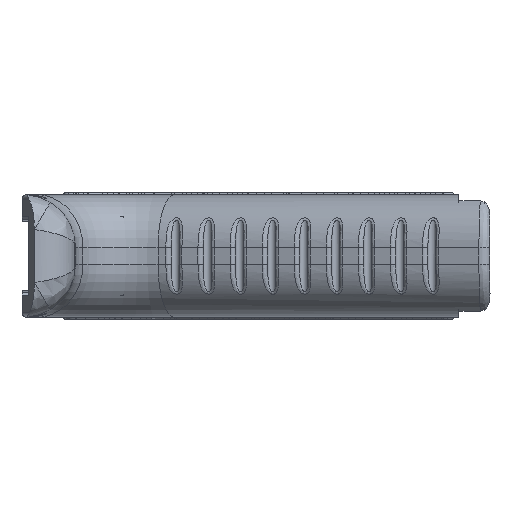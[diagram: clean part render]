
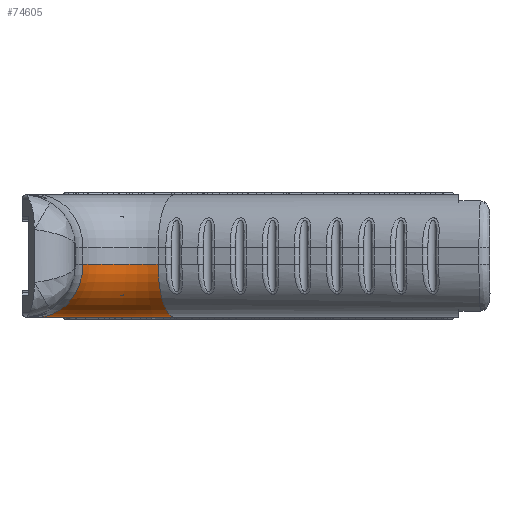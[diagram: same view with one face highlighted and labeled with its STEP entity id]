
A CAD part, left-side view. The second image highlights one B-rep face of the part: STEP entity #74605.
In plain terms, the highlighted toroidal (fillet/blend) face has major radius 27.537 mm and minor radius 12.5 mm.
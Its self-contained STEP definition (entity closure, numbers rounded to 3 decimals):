
#4588=TOROIDAL_SURFACE('',#77539,27.537,12.5);
#25821=FACE_OUTER_BOUND('',#30183,.T.);
#30183=EDGE_LOOP('',(#69851,#69852,#69853,#69854));
#30486=B_SPLINE_CURVE_WITH_KNOTS('',3,(#138049,#138050,#138051,#138052,
#138053,#138054,#138055,#138056,#138057,#138058,#138059,#138060,#138061,
#138062,#138063,#138064,#138065,#138066,#138067,#138068,#138069,#138070,
#138071,#138072,#138073,#138074,#138075,#138076,#138077,#138078,#138079,
#138080,#138081,#138082,#138083,#138084,#138085,#138086,#138087,#138088,
#138089,#138090,#138091,#138092,#138093,#138094,#138095,#138096,#138097,
#138098,#138099,#138100),.UNSPECIFIED.,.F.,.F.,(4,3,3,3,3,3,3,3,3,3,3,3,
3,3,3,3,3,4),(-0.008,0.,0.131,0.314,
0.448,0.497,0.627,0.806,
0.94,0.985,1.115,1.294,1.429,
1.473,1.604,1.783,1.915,1.961),
 .UNSPECIFIED.);
#30493=CIRCLE('',#74765,12.5);
#30698=CIRCLE('',#77131,27.537);
#30833=CIRCLE('',#77540,15.037);
#30883=VERTEX_POINT('',#91157);
#30884=VERTEX_POINT('',#91159);
#37329=VERTEX_POINT('',#134942);
#37802=VERTEX_POINT('',#138032);
#37991=EDGE_CURVE('',#30883,#30884,#30493,.T.);
#47823=EDGE_CURVE('',#37329,#30884,#30698,.T.);
#48535=EDGE_CURVE('',#37329,#37802,#30486,.T.);
#48566=EDGE_CURVE('',#30883,#37802,#30833,.T.);
#69851=ORIENTED_EDGE('',*,*,#47823,.T.);
#69852=ORIENTED_EDGE('',*,*,#37991,.F.);
#69853=ORIENTED_EDGE('',*,*,#48566,.T.);
#69854=ORIENTED_EDGE('',*,*,#48535,.F.);
#74605=ADVANCED_FACE('',(#25821),#4588,.T.);
#74765=AXIS2_PLACEMENT_3D('',#91160,#77754,#77755);
#77131=AXIS2_PLACEMENT_3D('',#134943,#88995,#88996);
#77539=AXIS2_PLACEMENT_3D('',#138200,#90288,#90289);
#77540=AXIS2_PLACEMENT_3D('',#138201,#90290,#90291);
#77754=DIRECTION('center_axis',(-0.309,-0.951,0.));
#77755=DIRECTION('ref_axis',(-0.951,0.309,0.));
#88995=DIRECTION('center_axis',(0.,0.,-1.));
#88996=DIRECTION('ref_axis',(0.93,0.368,0.));
#90288=DIRECTION('center_axis',(0.,0.,1.));
#90289=DIRECTION('ref_axis',(1.,0.,0.));
#90290=DIRECTION('center_axis',(0.,0.,1.));
#90291=DIRECTION('ref_axis',(0.93,0.368,0.));
#91157=CARTESIAN_POINT('',(-66.022,17.2,-21.5));
#91159=CARTESIAN_POINT('',(-54.134,13.337,-34.));
#91160=CARTESIAN_POINT('Origin',(-54.134,13.337,-21.5));
#134942=CARTESIAN_POINT('',(-66.871,45.874,-34.));
#134943=CARTESIAN_POINT('Origin',(-80.324,21.847,-34.));
#138032=CARTESIAN_POINT('',(-73.077,35.023,-21.5));
#138049=CARTESIAN_POINT('Ctrl Pts',(-66.871,45.874,
-34.));
#138050=CARTESIAN_POINT('Ctrl Pts',(-66.885,45.85,
-34.));
#138051=CARTESIAN_POINT('Ctrl Pts',(-66.899,45.826,
-34.));
#138052=CARTESIAN_POINT('Ctrl Pts',(-66.912,45.802,-34.));
#138053=CARTESIAN_POINT('Ctrl Pts',(-67.129,45.424,
-33.997));
#138054=CARTESIAN_POINT('Ctrl Pts',(-67.344,45.047,
-33.971));
#138055=CARTESIAN_POINT('Ctrl Pts',(-67.559,44.672,
-33.923));
#138056=CARTESIAN_POINT('Ctrl Pts',(-67.858,44.148,-33.856));
#138057=CARTESIAN_POINT('Ctrl Pts',(-68.155,43.629,-33.745));
#138058=CARTESIAN_POINT('Ctrl Pts',(-68.446,43.119,
-33.59));
#138059=CARTESIAN_POINT('Ctrl Pts',(-68.661,42.744,
-33.477));
#138060=CARTESIAN_POINT('Ctrl Pts',(-68.873,42.374,-33.34));
#138061=CARTESIAN_POINT('Ctrl Pts',(-69.08,42.01,
-33.181));
#138062=CARTESIAN_POINT('Ctrl Pts',(-69.155,41.88,
-33.124));
#138063=CARTESIAN_POINT('Ctrl Pts',(-69.229,41.751,
-33.064));
#138064=CARTESIAN_POINT('Ctrl Pts',(-69.302,41.622,-33.001));
#138065=CARTESIAN_POINT('Ctrl Pts',(-69.501,41.275,
-32.83));
#138066=CARTESIAN_POINT('Ctrl Pts',(-69.695,40.936,
-32.639));
#138067=CARTESIAN_POINT('Ctrl Pts',(-69.883,40.607,
-32.429));
#138068=CARTESIAN_POINT('Ctrl Pts',(-70.141,40.156,-32.14));
#138069=CARTESIAN_POINT('Ctrl Pts',(-70.388,39.724,
-31.815));
#138070=CARTESIAN_POINT('Ctrl Pts',(-70.623,39.313,
-31.456));
#138071=CARTESIAN_POINT('Ctrl Pts',(-70.799,39.005,
-31.187));
#138072=CARTESIAN_POINT('Ctrl Pts',(-70.969,38.709,
-30.898));
#138073=CARTESIAN_POINT('Ctrl Pts',(-71.13,38.427,
-30.591));
#138074=CARTESIAN_POINT('Ctrl Pts',(-71.184,38.333,
-30.489));
#138075=CARTESIAN_POINT('Ctrl Pts',(-71.236,38.241,
-30.386));
#138076=CARTESIAN_POINT('Ctrl Pts',(-71.288,38.15,
-30.28));
#138077=CARTESIAN_POINT('Ctrl Pts',(-71.44,37.885,-29.971));
#138078=CARTESIAN_POINT('Ctrl Pts',(-71.583,37.635,
-29.646));
#138079=CARTESIAN_POINT('Ctrl Pts',(-71.717,37.4,
-29.308));
#138080=CARTESIAN_POINT('Ctrl Pts',(-71.901,37.078,
-28.844));
#138081=CARTESIAN_POINT('Ctrl Pts',(-72.069,36.785,
-28.354));
#138082=CARTESIAN_POINT('Ctrl Pts',(-72.219,36.523,
-27.842));
#138083=CARTESIAN_POINT('Ctrl Pts',(-72.332,36.326,
-27.456));
#138084=CARTESIAN_POINT('Ctrl Pts',(-72.435,36.146,
-27.057));
#138085=CARTESIAN_POINT('Ctrl Pts',(-72.527,35.985,
-26.647));
#138086=CARTESIAN_POINT('Ctrl Pts',(-72.556,35.933,
-26.514));
#138087=CARTESIAN_POINT('Ctrl Pts',(-72.585,35.883,
-26.38));
#138088=CARTESIAN_POINT('Ctrl Pts',(-72.613,35.835,
-26.245));
#138089=CARTESIAN_POINT('Ctrl Pts',(-72.695,35.691,
-25.841));
#138090=CARTESIAN_POINT('Ctrl Pts',(-72.767,35.566,
-25.429));
#138091=CARTESIAN_POINT('Ctrl Pts',(-72.827,35.46,-25.012));
#138092=CARTESIAN_POINT('Ctrl Pts',(-72.91,35.315,
-24.443));
#138093=CARTESIAN_POINT('Ctrl Pts',(-72.973,35.206,
-23.862));
#138094=CARTESIAN_POINT('Ctrl Pts',(-73.014,35.133,
-23.276));
#138095=CARTESIAN_POINT('Ctrl Pts',(-73.045,35.079,
-22.84));
#138096=CARTESIAN_POINT('Ctrl Pts',(-73.065,35.044,
-22.402));
#138097=CARTESIAN_POINT('Ctrl Pts',(-73.073,35.03,
-21.961));
#138098=CARTESIAN_POINT('Ctrl Pts',(-73.076,35.025,
-21.808));
#138099=CARTESIAN_POINT('Ctrl Pts',(-73.077,35.023,-21.654));
#138100=CARTESIAN_POINT('Ctrl Pts',(-73.077,35.023,-21.5));
#138200=CARTESIAN_POINT('Origin',(-80.324,21.847,-21.5));
#138201=CARTESIAN_POINT('Origin',(-80.324,21.847,-21.5));
